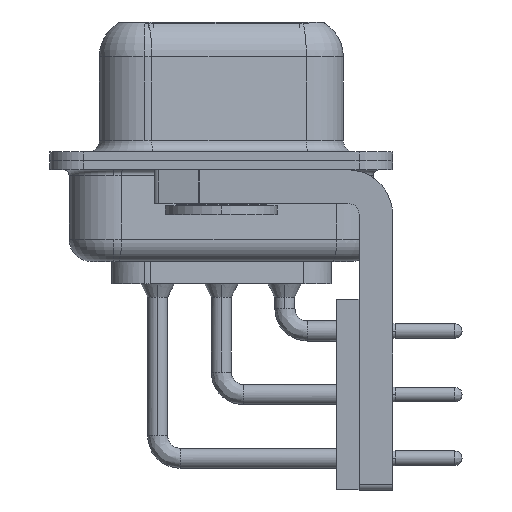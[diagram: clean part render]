
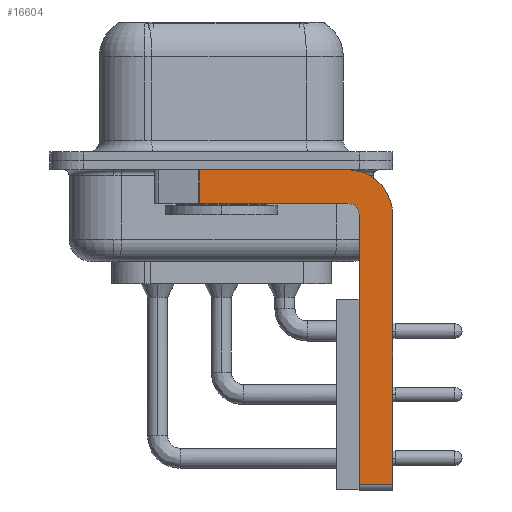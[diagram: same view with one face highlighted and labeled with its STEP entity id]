
A CAD part, left-side view. The second image highlights one B-rep face of the part: STEP entity #16604.
In plain terms, the highlighted planar face has unit normal (-1, 0, 0).
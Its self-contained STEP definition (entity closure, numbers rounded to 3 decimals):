
#174 = EDGE_CURVE ( 'NONE', #26578, #31306, #22906, .T. ) ;
#1136 = VECTOR ( 'NONE', #24473, 1000. ) ;
#1598 = CARTESIAN_POINT ( 'NONE',  ( -2.9, -7.65, -14.45 ) ) ;
#2486 = DIRECTION ( 'NONE',  ( 0., -1., 0. ) ) ;
#2762 = ORIENTED_EDGE ( 'NONE', *, *, #20688, .T. ) ;
#2932 = ORIENTED_EDGE ( 'NONE', *, *, #174, .F. ) ;
#3575 = ORIENTED_EDGE ( 'NONE', *, *, #32955, .F. ) ;
#3807 = CARTESIAN_POINT ( 'NONE',  ( -2.9, 3., -0.4 ) ) ;
#3861 = EDGE_CURVE ( 'NONE', #18188, #34107, #25056, .T. ) ;
#4382 = CARTESIAN_POINT ( 'NONE',  ( -2.9, -6.15, -2.4 ) ) ;
#6885 = ORIENTED_EDGE ( 'NONE', *, *, #3861, .F. ) ;
#7303 = CARTESIAN_POINT ( 'NONE',  ( -2.9, 0.978, -0.4 ) ) ;
#7459 = CARTESIAN_POINT ( 'NONE',  ( -2.9, -5.65, -2.4 ) ) ;
#7698 = CARTESIAN_POINT ( 'NONE',  ( -2.9, -6.15, -14.45 ) ) ;
#7730 = CARTESIAN_POINT ( 'NONE',  ( -2.9, -7.65, -2.4 ) ) ;
#8782 = LINE ( 'NONE', #19176, #22672 ) ;
#9304 = VECTOR ( 'NONE', #15560, 1000. ) ;
#9808 = EDGE_CURVE ( 'NONE', #31306, #16310, #35674, .T. ) ;
#10237 = EDGE_CURVE ( 'NONE', #21603, #13024, #32477, .T. ) ;
#10372 = ORIENTED_EDGE ( 'NONE', *, *, #10237, .F. ) ;
#10473 = DIRECTION ( 'NONE',  ( 0., 0., -1. ) ) ;
#10596 = DIRECTION ( 'NONE',  ( 0., 0., -1. ) ) ;
#10700 = DIRECTION ( 'NONE',  ( -1., 0., 0. ) ) ;
#10737 = EDGE_CURVE ( 'NONE', #21603, #37213, #20521, .T. ) ;
#11270 = CARTESIAN_POINT ( 'NONE',  ( -2.9, -5.65, -14.45 ) ) ;
#12478 = CIRCLE ( 'NONE', #28359, 2. ) ;
#13024 = VERTEX_POINT ( 'NONE', #23513 ) ;
#13802 = AXIS2_PLACEMENT_3D ( 'NONE', #36950, #28248, #10596 ) ;
#14295 = CARTESIAN_POINT ( 'NONE',  ( -2.9, -5.65, -1.9 ) ) ;
#14599 = AXIS2_PLACEMENT_3D ( 'NONE', #28355, #10700, #31321 ) ;
#14620 = CARTESIAN_POINT ( 'NONE',  ( -2.9, -7.65, -2.4 ) ) ;
#15560 = DIRECTION ( 'NONE',  ( 0., 0., -1. ) ) ;
#16310 = VERTEX_POINT ( 'NONE', #14295 ) ;
#16561 = EDGE_CURVE ( 'NONE', #13024, #18188, #12478, .T. ) ;
#16604 = ADVANCED_FACE ( 'NONE', ( #27236 ), #31109, .F. ) ;
#17702 = LINE ( 'NONE', #11270, #24609 ) ;
#17975 = CARTESIAN_POINT ( 'NONE',  ( -2.9, -6.15, -14.7 ) ) ;
#18188 = VERTEX_POINT ( 'NONE', #7730 ) ;
#19176 = CARTESIAN_POINT ( 'NONE',  ( -2.9, -5.65, -1.9 ) ) ;
#19250 = ORIENTED_EDGE ( 'NONE', *, *, #9808, .F. ) ;
#20518 = DIRECTION ( 'NONE',  ( 0., 0., 1. ) ) ;
#20521 = LINE ( 'NONE', #21680, #26485 ) ;
#20688 = EDGE_CURVE ( 'NONE', #26578, #34107, #17702, .T. ) ;
#21603 = VERTEX_POINT ( 'NONE', #7303 ) ;
#21680 = CARTESIAN_POINT ( 'NONE',  ( -2.9, 0.978, -1.9 ) ) ;
#22611 = CARTESIAN_POINT ( 'NONE',  ( -2.9, 0.978, -1.9 ) ) ;
#22672 = VECTOR ( 'NONE', #25072, 1000. ) ;
#22906 = LINE ( 'NONE', #17975, #31663 ) ;
#23513 = CARTESIAN_POINT ( 'NONE',  ( -2.9, -5.65, -0.4 ) ) ;
#24473 = DIRECTION ( 'NONE',  ( 0., -1., 0. ) ) ;
#24609 = VECTOR ( 'NONE', #2486, 1000. ) ;
#25056 = LINE ( 'NONE', #14620, #9304 ) ;
#25072 = DIRECTION ( 'NONE',  ( 0., 1., 0. ) ) ;
#26485 = VECTOR ( 'NONE', #30569, 1000. ) ;
#26578 = VERTEX_POINT ( 'NONE', #7698 ) ;
#27118 = EDGE_LOOP ( 'NONE', ( #10372, #34128, #3575, #19250, #2932, #2762, #6885, #31830 ) ) ;
#27236 = FACE_OUTER_BOUND ( 'NONE', #27118, .T. ) ;
#28124 = DIRECTION ( 'NONE',  ( 1., 0., 0. ) ) ;
#28248 = DIRECTION ( 'NONE',  ( 1., 0., 0. ) ) ;
#28355 = CARTESIAN_POINT ( 'NONE',  ( -2.9, -5.65, -2.4 ) ) ;
#28359 = AXIS2_PLACEMENT_3D ( 'NONE', #7459, #28124, #10473 ) ;
#30569 = DIRECTION ( 'NONE',  ( 0., 0., -1. ) ) ;
#31109 = PLANE ( 'NONE',  #13802 ) ;
#31306 = VERTEX_POINT ( 'NONE', #4382 ) ;
#31321 = DIRECTION ( 'NONE',  ( 0., 0., 1. ) ) ;
#31663 = VECTOR ( 'NONE', #20518, 1000. ) ;
#31830 = ORIENTED_EDGE ( 'NONE', *, *, #16561, .F. ) ;
#32477 = LINE ( 'NONE', #3807, #1136 ) ;
#32955 = EDGE_CURVE ( 'NONE', #16310, #37213, #8782, .T. ) ;
#34107 = VERTEX_POINT ( 'NONE', #1598 ) ;
#34128 = ORIENTED_EDGE ( 'NONE', *, *, #10737, .T. ) ;
#35674 = CIRCLE ( 'NONE', #14599, 0.5 ) ;
#36950 = CARTESIAN_POINT ( 'NONE',  ( -2.9, -5.65, -2.4 ) ) ;
#37213 = VERTEX_POINT ( 'NONE', #22611 ) ;
